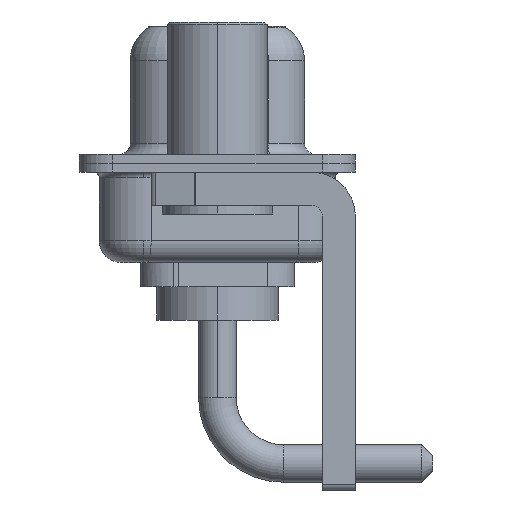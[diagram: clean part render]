
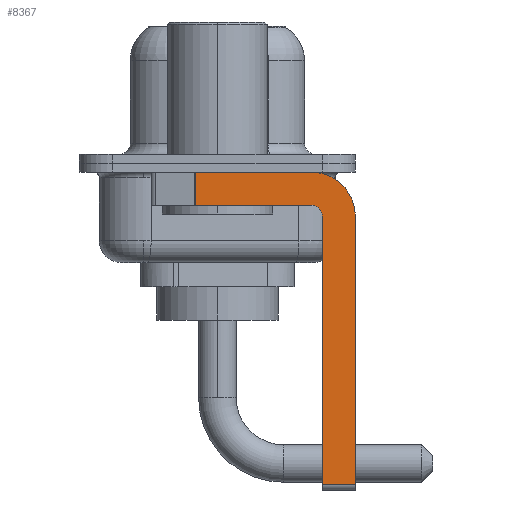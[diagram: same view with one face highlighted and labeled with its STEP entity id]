
A CAD part, left-side view. The second image highlights one B-rep face of the part: STEP entity #8367.
In plain terms, the highlighted planar face has unit normal (-1, 0, 0).
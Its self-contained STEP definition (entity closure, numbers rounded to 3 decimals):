
#9 = CARTESIAN_POINT ( 'NONE',  ( -2.9, -4.25, -2.4 ) ) ;
#102 = DIRECTION ( 'NONE',  ( -1., 0., 0. ) ) ;
#418 = LINE ( 'NONE', #5250, #12759 ) ;
#440 = CARTESIAN_POINT ( 'NONE',  ( -2.9, -6.25, -2.4 ) ) ;
#650 = DIRECTION ( 'NONE',  ( 1., 0., 0. ) ) ;
#836 = ORIENTED_EDGE ( 'NONE', *, *, #9801, .F. ) ;
#1395 = CARTESIAN_POINT ( 'NONE',  ( -2.9, 3., -0.4 ) ) ;
#1533 = CARTESIAN_POINT ( 'NONE',  ( -2.9, -4.75, -14.55 ) ) ;
#1627 = EDGE_CURVE ( 'NONE', #1630, #9312, #7242, .T. ) ;
#1630 = VERTEX_POINT ( 'NONE', #14657 ) ;
#1718 = VERTEX_POINT ( 'NONE', #1533 ) ;
#1908 = VERTEX_POINT ( 'NONE', #11649 ) ;
#2101 = ORIENTED_EDGE ( 'NONE', *, *, #14952, .T. ) ;
#2246 = DIRECTION ( 'NONE',  ( 0., -1., 0. ) ) ;
#2558 = LINE ( 'NONE', #1395, #5904 ) ;
#2637 = VERTEX_POINT ( 'NONE', #440 ) ;
#3049 = EDGE_CURVE ( 'NONE', #11355, #1908, #2558, .T. ) ;
#3576 = AXIS2_PLACEMENT_3D ( 'NONE', #9, #102, #4840 ) ;
#3615 = ORIENTED_EDGE ( 'NONE', *, *, #3049, .F. ) ;
#3907 = DIRECTION ( 'NONE',  ( 0., 0., -1. ) ) ;
#4340 = AXIS2_PLACEMENT_3D ( 'NONE', #10095, #7531, #7452 ) ;
#4498 = CARTESIAN_POINT ( 'NONE',  ( -2.9, -4.25, -2.4 ) ) ;
#4690 = VERTEX_POINT ( 'NONE', #12392 ) ;
#4714 = CARTESIAN_POINT ( 'NONE',  ( -2.9, -4.25, -14.55 ) ) ;
#4840 = DIRECTION ( 'NONE',  ( 0., 0., 1. ) ) ;
#5090 = CIRCLE ( 'NONE', #3576, 0.5 ) ;
#5250 = CARTESIAN_POINT ( 'NONE',  ( -2.9, 0.978, -1.9 ) ) ;
#5371 = PLANE ( 'NONE',  #4340 ) ;
#5417 = CARTESIAN_POINT ( 'NONE',  ( -2.9, -6.25, -2.4 ) ) ;
#5426 = VECTOR ( 'NONE', #6040, 1000. ) ;
#5428 = LINE ( 'NONE', #6699, #15170 ) ;
#5690 = EDGE_CURVE ( 'NONE', #1718, #8593, #5428, .T. ) ;
#5904 = VECTOR ( 'NONE', #2246, 1000. ) ;
#5997 = ORIENTED_EDGE ( 'NONE', *, *, #5690, .F. ) ;
#6040 = DIRECTION ( 'NONE',  ( 0., 1., 0. ) ) ;
#6699 = CARTESIAN_POINT ( 'NONE',  ( -2.9, -4.75, -14.8 ) ) ;
#7233 = EDGE_CURVE ( 'NONE', #1718, #4690, #10944, .T. ) ;
#7242 = LINE ( 'NONE', #12160, #5426 ) ;
#7386 = CARTESIAN_POINT ( 'NONE',  ( -2.9, 0.978, -1.9 ) ) ;
#7452 = DIRECTION ( 'NONE',  ( 0., 0., -1. ) ) ;
#7489 = VECTOR ( 'NONE', #11928, 1000. ) ;
#7531 = DIRECTION ( 'NONE',  ( 1., 0., 0. ) ) ;
#7748 = ORIENTED_EDGE ( 'NONE', *, *, #1627, .F. ) ;
#8169 = DIRECTION ( 'NONE',  ( 0., 0., -1. ) ) ;
#8367 = ADVANCED_FACE ( 'NONE', ( #9056 ), #5371, .F. ) ;
#8593 = VERTEX_POINT ( 'NONE', #13149 ) ;
#8984 = ORIENTED_EDGE ( 'NONE', *, *, #13714, .F. ) ;
#9056 = FACE_OUTER_BOUND ( 'NONE', #15053, .T. ) ;
#9095 = DIRECTION ( 'NONE',  ( 0., 0., 1. ) ) ;
#9312 = VERTEX_POINT ( 'NONE', #7386 ) ;
#9363 = EDGE_CURVE ( 'NONE', #8593, #1630, #5090, .T. ) ;
#9423 = CIRCLE ( 'NONE', #13030, 2. ) ;
#9801 = EDGE_CURVE ( 'NONE', #1908, #2637, #9423, .T. ) ;
#10095 = CARTESIAN_POINT ( 'NONE',  ( -2.9, -4.25, -2.4 ) ) ;
#10277 = VECTOR ( 'NONE', #12713, 1000. ) ;
#10944 = LINE ( 'NONE', #4714, #7489 ) ;
#11355 = VERTEX_POINT ( 'NONE', #13917 ) ;
#11649 = CARTESIAN_POINT ( 'NONE',  ( -2.9, -4.25, -0.4 ) ) ;
#11928 = DIRECTION ( 'NONE',  ( 0., -1., 0. ) ) ;
#12160 = CARTESIAN_POINT ( 'NONE',  ( -2.9, -4.25, -1.9 ) ) ;
#12392 = CARTESIAN_POINT ( 'NONE',  ( -2.9, -6.25, -14.55 ) ) ;
#12417 = ORIENTED_EDGE ( 'NONE', *, *, #9363, .F. ) ;
#12433 = ORIENTED_EDGE ( 'NONE', *, *, #7233, .T. ) ;
#12555 = LINE ( 'NONE', #5417, #10277 ) ;
#12713 = DIRECTION ( 'NONE',  ( 0., 0., -1. ) ) ;
#12759 = VECTOR ( 'NONE', #3907, 1000. ) ;
#13030 = AXIS2_PLACEMENT_3D ( 'NONE', #4498, #650, #8169 ) ;
#13149 = CARTESIAN_POINT ( 'NONE',  ( -2.9, -4.75, -2.4 ) ) ;
#13714 = EDGE_CURVE ( 'NONE', #2637, #4690, #12555, .T. ) ;
#13917 = CARTESIAN_POINT ( 'NONE',  ( -2.9, 0.978, -0.4 ) ) ;
#14657 = CARTESIAN_POINT ( 'NONE',  ( -2.9, -4.25, -1.9 ) ) ;
#14952 = EDGE_CURVE ( 'NONE', #11355, #9312, #418, .T. ) ;
#15053 = EDGE_LOOP ( 'NONE', ( #3615, #2101, #7748, #12417, #5997, #12433, #8984, #836 ) ) ;
#15170 = VECTOR ( 'NONE', #9095, 1000. ) ;
